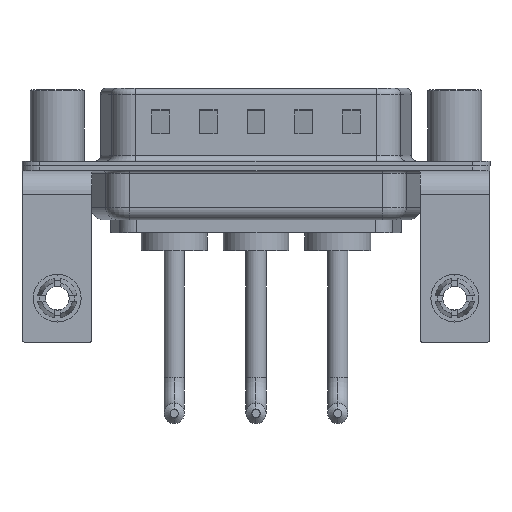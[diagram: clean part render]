
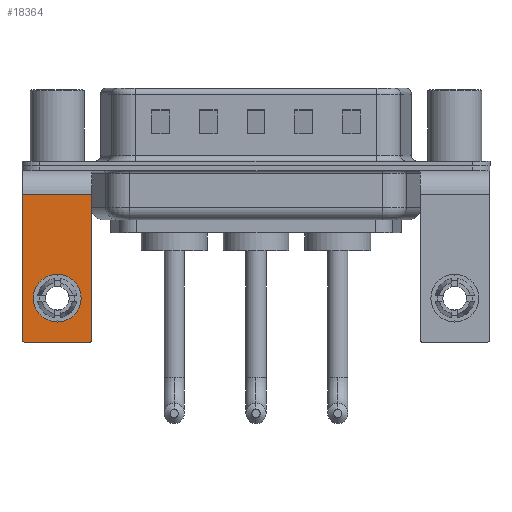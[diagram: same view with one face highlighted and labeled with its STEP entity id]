
A CAD part, front view. The second image highlights one B-rep face of the part: STEP entity #18364.
In plain terms, the highlighted planar face has unit normal (0, -1, 0).
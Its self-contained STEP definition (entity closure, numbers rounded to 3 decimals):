
#176 = CARTESIAN_POINT ( 'NONE',  ( 2.9, -6.25, -14.55 ) ) ;
#410 = AXIS2_PLACEMENT_3D ( 'NONE', #15727, #5086, #12405 ) ;
#947 = EDGE_CURVE ( 'NONE', #10776, #10976, #7871, .T. ) ;
#1629 = VERTEX_POINT ( 'NONE', #12913 ) ;
#1676 = CIRCLE ( 'NONE', #6787, 2. ) ;
#1818 = ORIENTED_EDGE ( 'NONE', *, *, #8528, .F. ) ;
#1821 = EDGE_CURVE ( 'NONE', #13058, #1629, #8720, .T. ) ;
#1874 = DIRECTION ( 'NONE',  ( -1., 0., 0. ) ) ;
#1984 = ORIENTED_EDGE ( 'NONE', *, *, #11638, .T. ) ;
#2247 = CIRCLE ( 'NONE', #12807, 0.25 ) ;
#2475 = EDGE_LOOP ( 'NONE', ( #10938, #12714, #1818, #1984, #16586, #14091 ) ) ;
#2896 = FACE_OUTER_BOUND ( 'NONE', #2475, .T. ) ;
#4107 = CARTESIAN_POINT ( 'NONE',  ( 2.65, -6.25, -14.55 ) ) ;
#4302 = VECTOR ( 'NONE', #5517, 1000. ) ;
#4446 = EDGE_CURVE ( 'NONE', #10776, #5454, #12367, .T. ) ;
#4516 = ORIENTED_EDGE ( 'NONE', *, *, #1821, .T. ) ;
#4541 = CARTESIAN_POINT ( 'NONE',  ( 2.65, -6.25, -14.8 ) ) ;
#4833 = CARTESIAN_POINT ( 'NONE',  ( -2.9, -6.25, -14.55 ) ) ;
#4953 = CARTESIAN_POINT ( 'NONE',  ( 2.9, -6.25, -2.4 ) ) ;
#5005 = ORIENTED_EDGE ( 'NONE', *, *, #15899, .T. ) ;
#5086 = DIRECTION ( 'NONE',  ( 0., 1., 0. ) ) ;
#5454 = VERTEX_POINT ( 'NONE', #176 ) ;
#5517 = DIRECTION ( 'NONE',  ( 0., 0., -1. ) ) ;
#5722 = CARTESIAN_POINT ( 'NONE',  ( -2.9, -6.25, -2.4 ) ) ;
#6002 = DIRECTION ( 'NONE',  ( 0., 0., 1. ) ) ;
#6287 = VERTEX_POINT ( 'NONE', #4833 ) ;
#6360 = CARTESIAN_POINT ( 'NONE',  ( 0., -6.25, -9.07 ) ) ;
#6413 = CIRCLE ( 'NONE', #17302, 0.25 ) ;
#6787 = AXIS2_PLACEMENT_3D ( 'NONE', #11905, #8808, #6002 ) ;
#7590 = VECTOR ( 'NONE', #1874, 1000. ) ;
#7603 = FACE_BOUND ( 'NONE', #11187, .T. ) ;
#7871 = LINE ( 'NONE', #8319, #17509 ) ;
#8319 = CARTESIAN_POINT ( 'NONE',  ( 2.9, -6.25, -2.4 ) ) ;
#8431 = VECTOR ( 'NONE', #16799, 1000. ) ;
#8528 = EDGE_CURVE ( 'NONE', #13558, #16903, #15634, .T. ) ;
#8720 = CIRCLE ( 'NONE', #410, 2. ) ;
#8808 = DIRECTION ( 'NONE',  ( 0., 1., 0. ) ) ;
#9614 = CARTESIAN_POINT ( 'NONE',  ( -2.65, -6.25, -14.8 ) ) ;
#9642 = CARTESIAN_POINT ( 'NONE',  ( -2.9, -6.25, -2.4 ) ) ;
#10205 = DIRECTION ( 'NONE',  ( 0., -1., 0. ) ) ;
#10776 = VERTEX_POINT ( 'NONE', #4953 ) ;
#10795 = CARTESIAN_POINT ( 'NONE',  ( -2.65, -6.25, -14.55 ) ) ;
#10938 = ORIENTED_EDGE ( 'NONE', *, *, #19657, .T. ) ;
#10976 = VERTEX_POINT ( 'NONE', #9642 ) ;
#11047 = CARTESIAN_POINT ( 'NONE',  ( 2.9, -6.25, -2.4 ) ) ;
#11187 = EDGE_LOOP ( 'NONE', ( #5005, #4516 ) ) ;
#11638 = EDGE_CURVE ( 'NONE', #13558, #5454, #6413, .T. ) ;
#11766 = EDGE_CURVE ( 'NONE', #6287, #16903, #2247, .T. ) ;
#11905 = CARTESIAN_POINT ( 'NONE',  ( 0., -6.25, -11.07 ) ) ;
#12367 = LINE ( 'NONE', #11047, #8431 ) ;
#12405 = DIRECTION ( 'NONE',  ( 0., 0., 1. ) ) ;
#12509 = DIRECTION ( 'NONE',  ( 0., 0., 1. ) ) ;
#12700 = CARTESIAN_POINT ( 'NONE',  ( 2.9, -6.25, -14.8 ) ) ;
#12714 = ORIENTED_EDGE ( 'NONE', *, *, #11766, .T. ) ;
#12807 = AXIS2_PLACEMENT_3D ( 'NONE', #10795, #18344, #12509 ) ;
#12913 = CARTESIAN_POINT ( 'NONE',  ( 0., -6.25, -13.07 ) ) ;
#13058 = VERTEX_POINT ( 'NONE', #6360 ) ;
#13321 = DIRECTION ( 'NONE',  ( 0., 0., 1. ) ) ;
#13558 = VERTEX_POINT ( 'NONE', #4541 ) ;
#13642 = DIRECTION ( 'NONE',  ( 0., 0., 1. ) ) ;
#13742 = CARTESIAN_POINT ( 'NONE',  ( 2.9, -6.25, -2.4 ) ) ;
#14091 = ORIENTED_EDGE ( 'NONE', *, *, #947, .T. ) ;
#15252 = PLANE ( 'NONE',  #18973 ) ;
#15634 = LINE ( 'NONE', #12700, #7590 ) ;
#15727 = CARTESIAN_POINT ( 'NONE',  ( 0., -6.25, -11.07 ) ) ;
#15899 = EDGE_CURVE ( 'NONE', #1629, #13058, #1676, .T. ) ;
#16051 = LINE ( 'NONE', #5722, #4302 ) ;
#16554 = DIRECTION ( 'NONE',  ( 0., 1., 0. ) ) ;
#16586 = ORIENTED_EDGE ( 'NONE', *, *, #4446, .F. ) ;
#16799 = DIRECTION ( 'NONE',  ( 0., 0., -1. ) ) ;
#16903 = VERTEX_POINT ( 'NONE', #9614 ) ;
#17302 = AXIS2_PLACEMENT_3D ( 'NONE', #4107, #10205, #13321 ) ;
#17509 = VECTOR ( 'NONE', #18954, 1000. ) ;
#18344 = DIRECTION ( 'NONE',  ( 0., -1., 0. ) ) ;
#18364 = ADVANCED_FACE ( 'NONE', ( #7603, #2896 ), #15252, .F. ) ;
#18954 = DIRECTION ( 'NONE',  ( -1., 0., 0. ) ) ;
#18973 = AXIS2_PLACEMENT_3D ( 'NONE', #13742, #16554, #13642 ) ;
#19657 = EDGE_CURVE ( 'NONE', #10976, #6287, #16051, .T. ) ;
